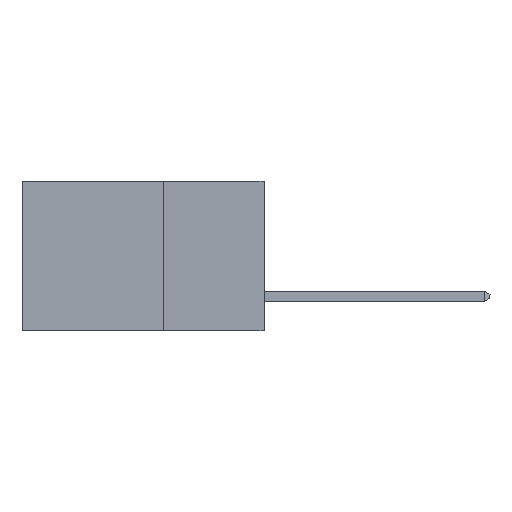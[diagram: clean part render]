
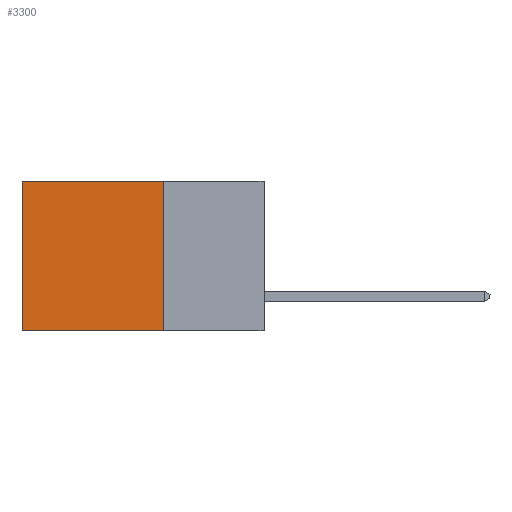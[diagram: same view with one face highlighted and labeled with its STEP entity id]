
A CAD part, left-side view. The second image highlights one B-rep face of the part: STEP entity #3300.
In plain terms, the highlighted planar face has unit normal (-1, 0, 0).
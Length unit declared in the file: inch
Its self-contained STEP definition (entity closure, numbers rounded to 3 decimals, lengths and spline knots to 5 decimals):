
#660 = LINE ( 'NONE', #6096, #673 ) ;
#673 = VECTOR ( 'NONE', #2235, 39.37008 ) ;
#884 = ORIENTED_EDGE ( 'NONE', *, *, #7495, .T. ) ;
#1200 = DIRECTION ( 'NONE',  ( 0., 0., -1. ) ) ;
#1330 = DIRECTION ( 'NONE',  ( 0., 1., 0. ) ) ;
#1340 = CARTESIAN_POINT ( 'NONE',  ( 0.2615, 0.25, 0. ) ) ;
#1376 = EDGE_CURVE ( 'NONE', #4225, #2611, #660, .T. ) ;
#2042 = VERTEX_POINT ( 'NONE', #6576 ) ;
#2156 = ORIENTED_EDGE ( 'NONE', *, *, #1376, .T. ) ;
#2223 = ORIENTED_EDGE ( 'NONE', *, *, #9147, .F. ) ;
#2235 = DIRECTION ( 'NONE',  ( 0., 0., -1. ) ) ;
#2611 = VERTEX_POINT ( 'NONE', #4348 ) ;
#2720 = CARTESIAN_POINT ( 'NONE',  ( 0.2615, 0.25, -0.37 ) ) ;
#3300 = ADVANCED_FACE ( 'NONE', ( #8157 ), #3486, .F. ) ;
#3486 = PLANE ( 'NONE',  #8315 ) ;
#3747 = EDGE_CURVE ( 'NONE', #8183, #2042, #5711, .T. ) ;
#4026 = EDGE_LOOP ( 'NONE', ( #2156, #2223, #5637, #884 ) ) ;
#4225 = VERTEX_POINT ( 'NONE', #9191 ) ;
#4348 = CARTESIAN_POINT ( 'NONE',  ( 0.2615, 0.6, -0.37 ) ) ;
#4620 = VECTOR ( 'NONE', #6157, 39.37008 ) ;
#4776 = VECTOR ( 'NONE', #1330, 39.37008 ) ;
#5072 = DIRECTION ( 'NONE',  ( 1., 0., 0. ) ) ;
#5215 = LINE ( 'NONE', #1340, #4620 ) ;
#5637 = ORIENTED_EDGE ( 'NONE', *, *, #3747, .F. ) ;
#5711 = LINE ( 'NONE', #7438, #7476 ) ;
#6096 = CARTESIAN_POINT ( 'NONE',  ( 0.2615, 0.6, -0.37 ) ) ;
#6157 = DIRECTION ( 'NONE',  ( 0., 1., 0. ) ) ;
#6576 = CARTESIAN_POINT ( 'NONE',  ( 0.2615, 0.25, -0.37 ) ) ;
#6759 = LINE ( 'NONE', #9852, #4776 ) ;
#7438 = CARTESIAN_POINT ( 'NONE',  ( 0.2615, 0.25, -0.37 ) ) ;
#7476 = VECTOR ( 'NONE', #9705, 39.37008 ) ;
#7495 = EDGE_CURVE ( 'NONE', #8183, #4225, #5215, .T. ) ;
#8157 = FACE_OUTER_BOUND ( 'NONE', #4026, .T. ) ;
#8183 = VERTEX_POINT ( 'NONE', #9035 ) ;
#8315 = AXIS2_PLACEMENT_3D ( 'NONE', #2720, #5072, #1200 ) ;
#9035 = CARTESIAN_POINT ( 'NONE',  ( 0.2615, 0.25, 0. ) ) ;
#9147 = EDGE_CURVE ( 'NONE', #2042, #2611, #6759, .T. ) ;
#9191 = CARTESIAN_POINT ( 'NONE',  ( 0.2615, 0.6, 0. ) ) ;
#9705 = DIRECTION ( 'NONE',  ( 0., 0., -1. ) ) ;
#9852 = CARTESIAN_POINT ( 'NONE',  ( 0.2615, 0.25, -0.37 ) ) ;
